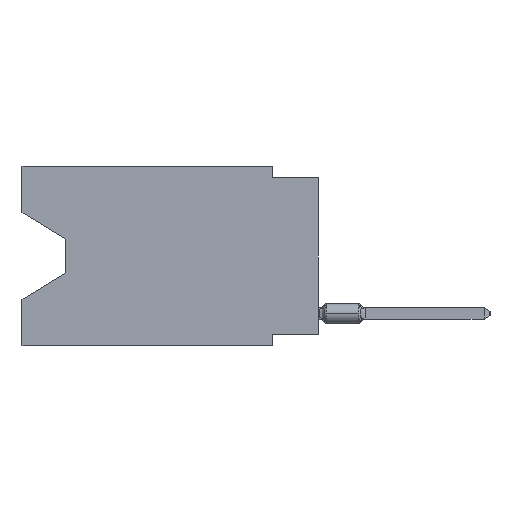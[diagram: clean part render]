
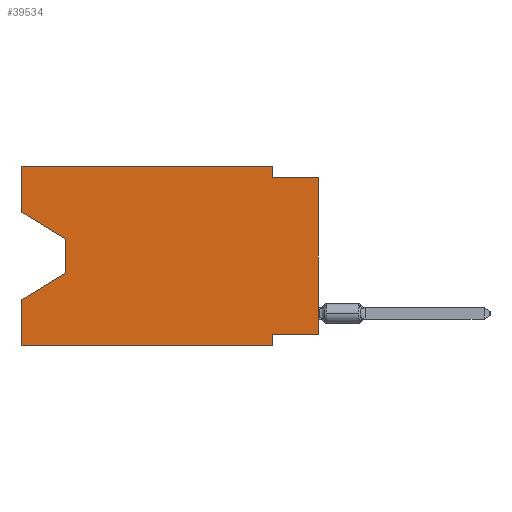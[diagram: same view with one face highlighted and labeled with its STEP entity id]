
A CAD part, left-side view. The second image highlights one B-rep face of the part: STEP entity #39534.
In plain terms, the highlighted planar face has unit normal (-1, 0, 0).
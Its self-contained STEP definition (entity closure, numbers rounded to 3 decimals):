
#1419 = CARTESIAN_POINT ( 'NONE',  ( 0., 0., 0. ) ) ;
#1492 = ORIENTED_EDGE ( 'NONE', *, *, #61933, .T. ) ;
#1951 = DIRECTION ( 'NONE',  ( 1., 0., 0. ) ) ;
#2017 = ORIENTED_EDGE ( 'NONE', *, *, #22093, .T. ) ;
#3083 = LINE ( 'NONE', #28150, #51788 ) ;
#3205 = LINE ( 'NONE', #77625, #45646 ) ;
#3358 = EDGE_CURVE ( 'NONE', #46811, #20238, #63461, .T. ) ;
#3511 = DIRECTION ( 'NONE',  ( 0., 0., 1. ) ) ;
#3594 = CARTESIAN_POINT ( 'NONE',  ( 0., 0., -0.635 ) ) ;
#4281 = CARTESIAN_POINT ( 'NONE',  ( 0., 16.383, 0. ) ) ;
#4434 = VECTOR ( 'NONE', #11459, 1000. ) ;
#6778 = LINE ( 'NONE', #50772, #33465 ) ;
#6947 = CARTESIAN_POINT ( 'NONE',  ( 0., 0., -0.635 ) ) ;
#7711 = PLANE ( 'NONE',  #73578 ) ;
#8260 = DIRECTION ( 'NONE',  ( 0., -1., 0. ) ) ;
#9448 = CARTESIAN_POINT ( 'NONE',  ( 0., 16.383, -2.546 ) ) ;
#11459 = DIRECTION ( 'NONE',  ( 0., 0., -1. ) ) ;
#11673 = CARTESIAN_POINT ( 'NONE',  ( 0., 13.97, -4.013 ) ) ;
#13694 = DIRECTION ( 'NONE',  ( 0., 0., -1. ) ) ;
#14352 = VECTOR ( 'NONE', #21750, 1000. ) ;
#14972 = DIRECTION ( 'NONE',  ( 0., 0., 1. ) ) ;
#15557 = EDGE_CURVE ( 'NONE', #48251, #46811, #67577, .T. ) ;
#20238 = VERTEX_POINT ( 'NONE', #78105 ) ;
#20846 = CARTESIAN_POINT ( 'NONE',  ( 0., 16.383, 0. ) ) ;
#21179 = CARTESIAN_POINT ( 'NONE',  ( 0., 16.383, -7.36 ) ) ;
#21750 = DIRECTION ( 'NONE',  ( 0., 0., -1. ) ) ;
#22093 = EDGE_CURVE ( 'NONE', #57314, #29327, #6778, .T. ) ;
#23897 = VERTEX_POINT ( 'NONE', #32969 ) ;
#24395 = ORIENTED_EDGE ( 'NONE', *, *, #58609, .T. ) ;
#26102 = DIRECTION ( 'NONE',  ( 0., 1., 0. ) ) ;
#26190 = VECTOR ( 'NONE', #8260, 1000. ) ;
#26493 = DIRECTION ( 'NONE',  ( 0., -0.855, -0.519 ) ) ;
#27942 = EDGE_CURVE ( 'NONE', #23897, #35224, #38839, .T. ) ;
#28150 = CARTESIAN_POINT ( 'NONE',  ( 0., 16.383, 0. ) ) ;
#28276 = DIRECTION ( 'NONE',  ( 0., 0.855, -0.519 ) ) ;
#29327 = VERTEX_POINT ( 'NONE', #11673 ) ;
#30118 = EDGE_CURVE ( 'NONE', #23897, #63396, #45389, .T. ) ;
#30184 = CARTESIAN_POINT ( 'NONE',  ( 0., 16.383, 0. ) ) ;
#31508 = ORIENTED_EDGE ( 'NONE', *, *, #33991, .F. ) ;
#32625 = VECTOR ( 'NONE', #26102, 1000. ) ;
#32969 = CARTESIAN_POINT ( 'NONE',  ( 0., 0., -9.271 ) ) ;
#33062 = CARTESIAN_POINT ( 'NONE',  ( 0., 0., -9.271 ) ) ;
#33465 = VECTOR ( 'NONE', #26493, 1000. ) ;
#33991 = EDGE_CURVE ( 'NONE', #52710, #61080, #3083, .T. ) ;
#34277 = ORIENTED_EDGE ( 'NONE', *, *, #38140, .F. ) ;
#35224 = VERTEX_POINT ( 'NONE', #54455 ) ;
#36397 = LINE ( 'NONE', #61916, #14352 ) ;
#37224 = EDGE_CURVE ( 'NONE', #52710, #79677, #39496, .T. ) ;
#37707 = CARTESIAN_POINT ( 'NONE',  ( 0., 16.383, 0. ) ) ;
#37716 = CARTESIAN_POINT ( 'NONE',  ( 0., 16.383, -9.906 ) ) ;
#38140 = EDGE_CURVE ( 'NONE', #35224, #79677, #36397, .T. ) ;
#38839 = LINE ( 'NONE', #33062, #32625 ) ;
#39115 = ORIENTED_EDGE ( 'NONE', *, *, #27942, .F. ) ;
#39496 = LINE ( 'NONE', #64608, #26190 ) ;
#39534 = ADVANCED_FACE ( 'NONE', ( #49266 ), #7711, .F. ) ;
#40169 = DIRECTION ( 'NONE',  ( 0., 0., -1. ) ) ;
#40458 = ORIENTED_EDGE ( 'NONE', *, *, #37224, .T. ) ;
#40590 = LINE ( 'NONE', #3594, #41177 ) ;
#40592 = VERTEX_POINT ( 'NONE', #50099 ) ;
#41177 = VECTOR ( 'NONE', #60727, 1000. ) ;
#42318 = VECTOR ( 'NONE', #79516, 1000. ) ;
#42509 = LINE ( 'NONE', #30184, #53464 ) ;
#44311 = LINE ( 'NONE', #81138, #4434 ) ;
#44440 = ORIENTED_EDGE ( 'NONE', *, *, #15557, .F. ) ;
#45389 = LINE ( 'NONE', #1419, #63010 ) ;
#45646 = VECTOR ( 'NONE', #28276, 1000. ) ;
#46594 = EDGE_LOOP ( 'NONE', ( #2017, #24395, #1492, #31508, #40458, #34277, #39115, #70490, #68007, #59224, #44440, #70665 ) ) ;
#46811 = VERTEX_POINT ( 'NONE', #57129 ) ;
#48251 = VERTEX_POINT ( 'NONE', #37707 ) ;
#49266 = FACE_OUTER_BOUND ( 'NONE', #46594, .T. ) ;
#50099 = CARTESIAN_POINT ( 'NONE',  ( 0., 13.97, -5.893 ) ) ;
#50772 = CARTESIAN_POINT ( 'NONE',  ( 0., 16.383, -2.546 ) ) ;
#51788 = VECTOR ( 'NONE', #59003, 1000. ) ;
#51811 = CARTESIAN_POINT ( 'NONE',  ( 0., 2.54, -9.906 ) ) ;
#51912 = CARTESIAN_POINT ( 'NONE',  ( 0., 2.54, 0. ) ) ;
#52710 = VERTEX_POINT ( 'NONE', #37716 ) ;
#53464 = VECTOR ( 'NONE', #3511, 1000. ) ;
#54455 = CARTESIAN_POINT ( 'NONE',  ( 0., 2.54, -9.271 ) ) ;
#57129 = CARTESIAN_POINT ( 'NONE',  ( 0., 2.54, 0. ) ) ;
#57314 = VERTEX_POINT ( 'NONE', #9448 ) ;
#58609 = EDGE_CURVE ( 'NONE', #29327, #40592, #44311, .T. ) ;
#58881 = EDGE_CURVE ( 'NONE', #20238, #63396, #40590, .T. ) ;
#59003 = DIRECTION ( 'NONE',  ( 0., 0., 1. ) ) ;
#59224 = ORIENTED_EDGE ( 'NONE', *, *, #3358, .F. ) ;
#60727 = DIRECTION ( 'NONE',  ( 0., -1., 0. ) ) ;
#61080 = VERTEX_POINT ( 'NONE', #21179 ) ;
#61219 = EDGE_CURVE ( 'NONE', #57314, #48251, #42509, .T. ) ;
#61916 = CARTESIAN_POINT ( 'NONE',  ( 0., 2.54, -9.906 ) ) ;
#61933 = EDGE_CURVE ( 'NONE', #40592, #61080, #3205, .T. ) ;
#63010 = VECTOR ( 'NONE', #14972, 1000. ) ;
#63396 = VERTEX_POINT ( 'NONE', #6947 ) ;
#63461 = LINE ( 'NONE', #51912, #79818 ) ;
#64608 = CARTESIAN_POINT ( 'NONE',  ( 0., 16.383, -9.906 ) ) ;
#67577 = LINE ( 'NONE', #4281, #42318 ) ;
#68007 = ORIENTED_EDGE ( 'NONE', *, *, #58881, .F. ) ;
#70490 = ORIENTED_EDGE ( 'NONE', *, *, #30118, .T. ) ;
#70665 = ORIENTED_EDGE ( 'NONE', *, *, #61219, .F. ) ;
#73578 = AXIS2_PLACEMENT_3D ( 'NONE', #20846, #1951, #40169 ) ;
#77625 = CARTESIAN_POINT ( 'NONE',  ( 0., 13.97, -5.893 ) ) ;
#78105 = CARTESIAN_POINT ( 'NONE',  ( 0., 2.54, -0.635 ) ) ;
#79516 = DIRECTION ( 'NONE',  ( 0., -1., 0. ) ) ;
#79677 = VERTEX_POINT ( 'NONE', #51811 ) ;
#79818 = VECTOR ( 'NONE', #13694, 1000. ) ;
#81138 = CARTESIAN_POINT ( 'NONE',  ( 0., 13.97, -4.013 ) ) ;
